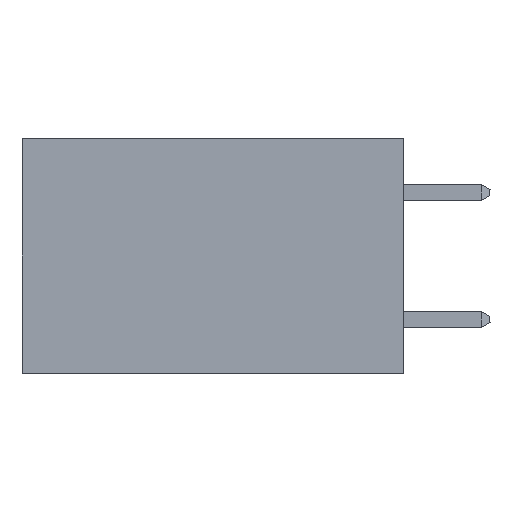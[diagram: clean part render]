
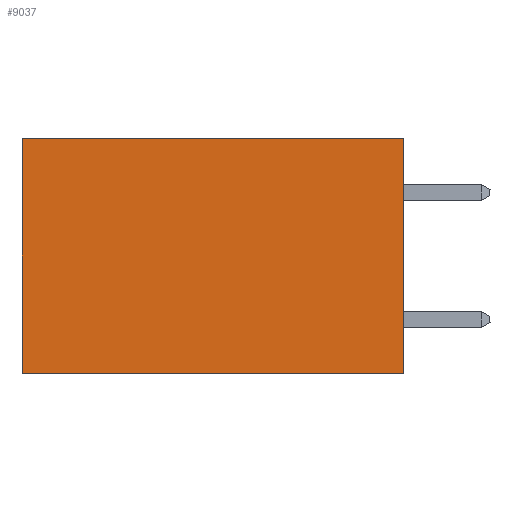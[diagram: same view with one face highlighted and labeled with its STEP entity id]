
A CAD part, left-side view. The second image highlights one B-rep face of the part: STEP entity #9037.
In plain terms, the highlighted planar face has unit normal (-1, 0, 0).
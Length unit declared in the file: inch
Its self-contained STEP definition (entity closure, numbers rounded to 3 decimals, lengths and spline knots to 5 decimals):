
#414 = CARTESIAN_POINT ( 'NONE',  ( 0.2875, 0., 0. ) ) ;
#482 = DIRECTION ( 'NONE',  ( 0., 1., 0. ) ) ;
#1371 = DIRECTION ( 'NONE',  ( 0., 0., -1. ) ) ;
#1626 = CARTESIAN_POINT ( 'NONE',  ( 0.2875, 0.6, -0.37 ) ) ;
#1735 = DIRECTION ( 'NONE',  ( 1., 0., 0. ) ) ;
#1828 = PLANE ( 'NONE',  #7140 ) ;
#1845 = EDGE_CURVE ( 'NONE', #21968, #25542, #20723, .T. ) ;
#2051 = CARTESIAN_POINT ( 'NONE',  ( 0.2875, 0., 0. ) ) ;
#2488 = VECTOR ( 'NONE', #482, 39.37008 ) ;
#4028 = DIRECTION ( 'NONE',  ( 0., 0., -1. ) ) ;
#5339 = EDGE_CURVE ( 'NONE', #23446, #12040, #8613, .T. ) ;
#5952 = CARTESIAN_POINT ( 'NONE',  ( 0.2875, 0.6, 0. ) ) ;
#7140 = AXIS2_PLACEMENT_3D ( 'NONE', #8202, #1735, #4028 ) ;
#8202 = CARTESIAN_POINT ( 'NONE',  ( 0.2875, 0., 0. ) ) ;
#8443 = VECTOR ( 'NONE', #17353, 39.37008 ) ;
#8484 = CARTESIAN_POINT ( 'NONE',  ( 0.2875, 0., 0. ) ) ;
#8613 = LINE ( 'NONE', #5952, #15435 ) ;
#9037 = ADVANCED_FACE ( 'NONE', ( #13897 ), #1828, .F. ) ;
#9330 = CARTESIAN_POINT ( 'NONE',  ( 0.2875, 0., -0.37 ) ) ;
#11405 = ORIENTED_EDGE ( 'NONE', *, *, #27394, .F. ) ;
#12040 = VERTEX_POINT ( 'NONE', #1626 ) ;
#12421 = ORIENTED_EDGE ( 'NONE', *, *, #25005, .T. ) ;
#12646 = ORIENTED_EDGE ( 'NONE', *, *, #1845, .F. ) ;
#13897 = FACE_OUTER_BOUND ( 'NONE', #15221, .T. ) ;
#14061 = LINE ( 'NONE', #9330, #2488 ) ;
#15221 = EDGE_LOOP ( 'NONE', ( #23702, #11405, #12646, #12421 ) ) ;
#15435 = VECTOR ( 'NONE', #1371, 39.37008 ) ;
#17094 = DIRECTION ( 'NONE',  ( 0., 1., 0. ) ) ;
#17353 = DIRECTION ( 'NONE',  ( 0., 0., -1. ) ) ;
#17992 = VECTOR ( 'NONE', #17094, 39.37008 ) ;
#18332 = CARTESIAN_POINT ( 'NONE',  ( 0.2875, 0.6, 0. ) ) ;
#20000 = CARTESIAN_POINT ( 'NONE',  ( 0.2875, 0., -0.37 ) ) ;
#20723 = LINE ( 'NONE', #8484, #8443 ) ;
#21968 = VERTEX_POINT ( 'NONE', #414 ) ;
#23446 = VERTEX_POINT ( 'NONE', #18332 ) ;
#23702 = ORIENTED_EDGE ( 'NONE', *, *, #5339, .T. ) ;
#24792 = LINE ( 'NONE', #2051, #17992 ) ;
#25005 = EDGE_CURVE ( 'NONE', #21968, #23446, #24792, .T. ) ;
#25542 = VERTEX_POINT ( 'NONE', #20000 ) ;
#27394 = EDGE_CURVE ( 'NONE', #25542, #12040, #14061, .T. ) ;
